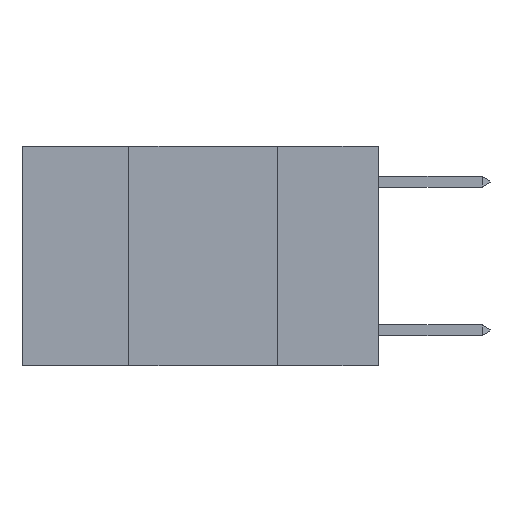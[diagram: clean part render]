
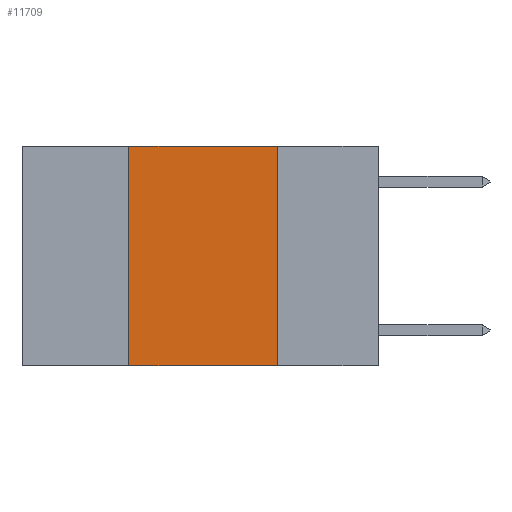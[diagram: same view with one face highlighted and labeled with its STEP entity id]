
A CAD part, left-side view. The second image highlights one B-rep face of the part: STEP entity #11709.
In plain terms, the highlighted planar face has unit normal (-1, 0, 0).
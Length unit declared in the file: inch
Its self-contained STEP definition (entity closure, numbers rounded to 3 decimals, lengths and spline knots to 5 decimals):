
#323 = DIRECTION ( 'NONE',  ( 0., -1., 0. ) ) ;
#695 = DIRECTION ( 'NONE',  ( 0., 0., -1. ) ) ;
#847 = LINE ( 'NONE', #19576, #4104 ) ;
#988 = ORIENTED_EDGE ( 'NONE', *, *, #6145, .F. ) ;
#2187 = CARTESIAN_POINT ( 'NONE',  ( 0., 0.6, -0.37 ) ) ;
#2347 = LINE ( 'NONE', #19222, #10775 ) ;
#2724 = FACE_OUTER_BOUND ( 'NONE', #8371, .T. ) ;
#3238 = VERTEX_POINT ( 'NONE', #14155 ) ;
#3520 = EDGE_CURVE ( 'NONE', #8890, #3238, #16949, .T. ) ;
#3794 = DIRECTION ( 'NONE',  ( 0., -1., 0. ) ) ;
#3905 = VECTOR ( 'NONE', #3794, 39.37008 ) ;
#4104 = VECTOR ( 'NONE', #695, 39.37008 ) ;
#4814 = VECTOR ( 'NONE', #8007, 39.37008 ) ;
#5288 = ORIENTED_EDGE ( 'NONE', *, *, #14970, .F. ) ;
#6145 = EDGE_CURVE ( 'NONE', #10322, #10872, #2347, .T. ) ;
#6246 = ORIENTED_EDGE ( 'NONE', *, *, #8441, .F. ) ;
#6396 = DIRECTION ( 'NONE',  ( 0., 0., -1. ) ) ;
#7947 = CARTESIAN_POINT ( 'NONE',  ( 0., 0.42, 0. ) ) ;
#8007 = DIRECTION ( 'NONE',  ( 0., 0., 1. ) ) ;
#8371 = EDGE_LOOP ( 'NONE', ( #5288, #988, #6246, #9163 ) ) ;
#8441 = EDGE_CURVE ( 'NONE', #8890, #10322, #13138, .T. ) ;
#8521 = AXIS2_PLACEMENT_3D ( 'NONE', #9430, #15788, #6396 ) ;
#8890 = VERTEX_POINT ( 'NONE', #13631 ) ;
#9163 = ORIENTED_EDGE ( 'NONE', *, *, #3520, .T. ) ;
#9430 = CARTESIAN_POINT ( 'NONE',  ( 0., 0.6, 0. ) ) ;
#10322 = VERTEX_POINT ( 'NONE', #18137 ) ;
#10775 = VECTOR ( 'NONE', #323, 39.37008 ) ;
#10872 = VERTEX_POINT ( 'NONE', #14801 ) ;
#11709 = ADVANCED_FACE ( 'NONE', ( #2724 ), #12604, .F. ) ;
#12604 = PLANE ( 'NONE',  #8521 ) ;
#13138 = LINE ( 'NONE', #7947, #4814 ) ;
#13631 = CARTESIAN_POINT ( 'NONE',  ( 0., 0.42, -0.37 ) ) ;
#14155 = CARTESIAN_POINT ( 'NONE',  ( 0., 0.17, -0.37 ) ) ;
#14801 = CARTESIAN_POINT ( 'NONE',  ( 0., 0.17, 0. ) ) ;
#14970 = EDGE_CURVE ( 'NONE', #10872, #3238, #847, .T. ) ;
#15788 = DIRECTION ( 'NONE',  ( 1., 0., 0. ) ) ;
#16949 = LINE ( 'NONE', #2187, #3905 ) ;
#18137 = CARTESIAN_POINT ( 'NONE',  ( 0., 0.42, 0. ) ) ;
#19222 = CARTESIAN_POINT ( 'NONE',  ( 0., 0.6, 0. ) ) ;
#19576 = CARTESIAN_POINT ( 'NONE',  ( 0., 0.17, 0. ) ) ;
